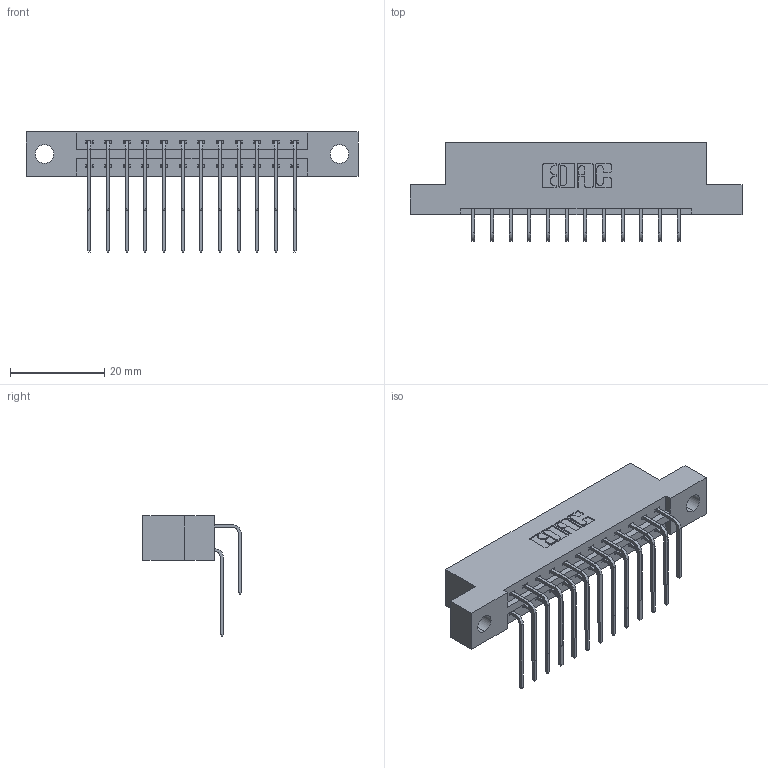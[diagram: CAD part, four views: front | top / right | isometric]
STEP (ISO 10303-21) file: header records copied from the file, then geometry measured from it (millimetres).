
FILE_DESCRIPTION (( 'STEP AP203' ), '1' );
FILE_NAME ('337-024-559-204.STEP', '2019-10-08T15:46:25', ( '' ), ( '' ), 'SwSTEP 2.0', 'SolidWorks 2016', '' );
FILE_SCHEMA (( 'CONFIG_CONTROL_DESIGN' ));
Length unit declared in the file: inch
Products named in the file (4): 345-292-001_559 Tail - 2; 345-292-001_558 559 Tail - 1; 337-024-559-204; 337 Part_Flush Mounting Lugs - 0.156 Dia-TH
Assembly tree (25 placements, depth 2):
  337-024-559-204
    337 Part_Flush Mounting Lugs - 0.156 Dia-TH
    345-292-001_558 559 Tail - 1  x12
    345-292-001_559 Tail - 2  x12
Bounding box: 70.56 x 20.9 x 25.53 mm (x, y, z)
Volume: 7087.6 mm3; surface area: 8213.7 mm2
Topology: 25 solids, 25 shells, 1458 faces, 4319 edges, 2846 vertices
Faces by surface type: plane 1030, cylinder 428
Entity records: 14971 total; most frequent: CARTESIAN_POINT 2593, ORIENTED_EDGE 2478, DIRECTION 2243, EDGE_CURVE 1239, LINE 1071, VECTOR 1071, VERTEX_POINT 822, AXIS2_PLACEMENT_3D 586
